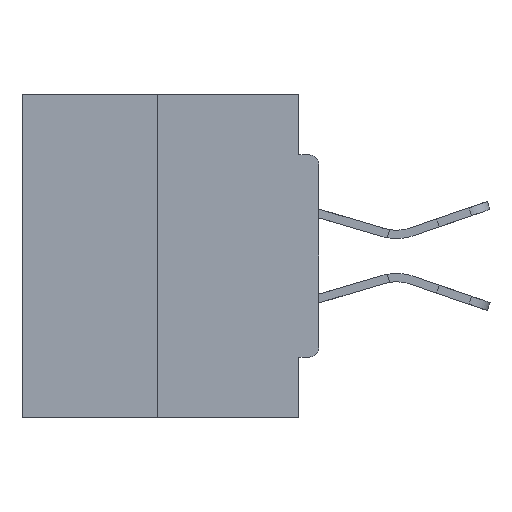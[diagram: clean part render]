
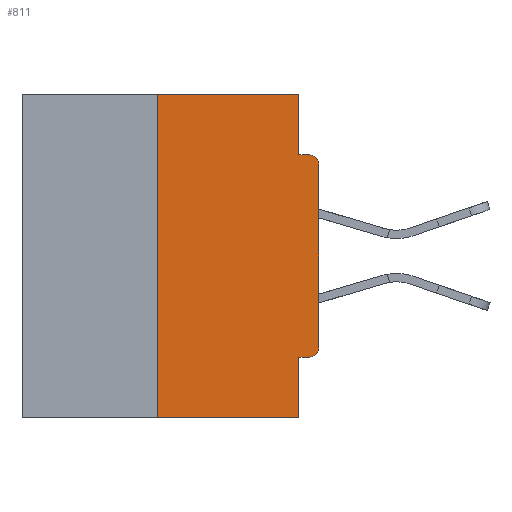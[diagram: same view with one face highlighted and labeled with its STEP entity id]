
A CAD part, left-side view. The second image highlights one B-rep face of the part: STEP entity #811.
In plain terms, the highlighted planar face has unit normal (-1, 0, 0).
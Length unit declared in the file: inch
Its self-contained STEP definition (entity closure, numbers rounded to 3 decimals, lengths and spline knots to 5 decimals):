
#811 = ADVANCED_FACE ( 'NONE', ( #11854 ), #10083, .F. ) ;
#915 = CARTESIAN_POINT ( 'NONE',  ( 0., 0.031, 0. ) ) ;
#2630 = AXIS2_PLACEMENT_3D ( 'NONE', #7279, #28383, #31005 ) ;
#3054 = LINE ( 'NONE', #5576, #21504 ) ;
#3866 = CARTESIAN_POINT ( 'NONE',  ( 0., 0.015, -0.4065 ) ) ;
#4381 = EDGE_CURVE ( 'NONE', #31245, #14231, #3054, .T. ) ;
#4686 = CARTESIAN_POINT ( 'NONE',  ( 0., 0.031, -0.4065 ) ) ;
#4790 = EDGE_CURVE ( 'NONE', #15706, #33267, #16122, .T. ) ;
#5576 = CARTESIAN_POINT ( 'NONE',  ( 0., 0., -0.0935 ) ) ;
#6225 = LINE ( 'NONE', #30858, #16854 ) ;
#6309 = DIRECTION ( 'NONE',  ( 0., 0., -1. ) ) ;
#6626 = DIRECTION ( 'NONE',  ( 0., -1., 0. ) ) ;
#7039 = VERTEX_POINT ( 'NONE', #24957 ) ;
#7138 = ORIENTED_EDGE ( 'NONE', *, *, #28937, .F. ) ;
#7237 = CARTESIAN_POINT ( 'NONE',  ( 0., 0.25, 0. ) ) ;
#7279 = CARTESIAN_POINT ( 'NONE',  ( 0., 0.015, -0.3915 ) ) ;
#7896 = DIRECTION ( 'NONE',  ( 0., 0., 1. ) ) ;
#8215 = VERTEX_POINT ( 'NONE', #30735 ) ;
#8433 = ORIENTED_EDGE ( 'NONE', *, *, #21307, .T. ) ;
#9488 = CARTESIAN_POINT ( 'NONE',  ( 0., 0.25, 0. ) ) ;
#9512 = VECTOR ( 'NONE', #22536, 39.37008 ) ;
#9720 = EDGE_CURVE ( 'NONE', #23108, #31245, #22672, .T. ) ;
#10083 = PLANE ( 'NONE',  #23533 ) ;
#10325 = CARTESIAN_POINT ( 'NONE',  ( 0., 0.015, -0.0935 ) ) ;
#10364 = DIRECTION ( 'NONE',  ( 0., -1., 0. ) ) ;
#11040 = ORIENTED_EDGE ( 'NONE', *, *, #19071, .T. ) ;
#11854 = FACE_OUTER_BOUND ( 'NONE', #15785, .T. ) ;
#12369 = DIRECTION ( 'NONE',  ( 0., 0., -1. ) ) ;
#13281 = VECTOR ( 'NONE', #18262, 39.37008 ) ;
#13799 = CARTESIAN_POINT ( 'NONE',  ( 0., 0., -0.1085 ) ) ;
#14213 = VERTEX_POINT ( 'NONE', #7237 ) ;
#14231 = VERTEX_POINT ( 'NONE', #10325 ) ;
#15110 = DIRECTION ( 'NONE',  ( 0., 0., -1. ) ) ;
#15706 = VERTEX_POINT ( 'NONE', #3866 ) ;
#15785 = EDGE_LOOP ( 'NONE', ( #24351, #17630, #11040, #7138, #28497, #24958, #16997, #8433, #25123, #32436 ) ) ;
#16122 = LINE ( 'NONE', #23552, #13281 ) ;
#16509 = CARTESIAN_POINT ( 'NONE',  ( 0., 0.015, -0.1085 ) ) ;
#16854 = VECTOR ( 'NONE', #15110, 39.37008 ) ;
#16997 = ORIENTED_EDGE ( 'NONE', *, *, #31982, .T. ) ;
#17535 = DIRECTION ( 'NONE',  ( 1., 0., 0. ) ) ;
#17630 = ORIENTED_EDGE ( 'NONE', *, *, #28107, .F. ) ;
#17719 = VECTOR ( 'NONE', #10364, 39.37008 ) ;
#18262 = DIRECTION ( 'NONE',  ( 0., 1., 0. ) ) ;
#19071 = EDGE_CURVE ( 'NONE', #27847, #7039, #24706, .T. ) ;
#19269 = DIRECTION ( 'NONE',  ( -1., 0., 0. ) ) ;
#20211 = EDGE_CURVE ( 'NONE', #14213, #23108, #24123, .T. ) ;
#20874 = VECTOR ( 'NONE', #6626, 39.37008 ) ;
#21179 = CARTESIAN_POINT ( 'NONE',  ( 0., 0.25, -0.5 ) ) ;
#21307 = EDGE_CURVE ( 'NONE', #25282, #14231, #23636, .T. ) ;
#21504 = VECTOR ( 'NONE', #26686, 39.37008 ) ;
#21807 = DIRECTION ( 'NONE',  ( 0., 0., -1. ) ) ;
#22213 = EDGE_CURVE ( 'NONE', #15706, #8215, #29349, .T. ) ;
#22536 = DIRECTION ( 'NONE',  ( 0., 0., 1. ) ) ;
#22672 = LINE ( 'NONE', #915, #28021 ) ;
#23108 = VERTEX_POINT ( 'NONE', #24574 ) ;
#23533 = AXIS2_PLACEMENT_3D ( 'NONE', #28099, #17535, #12369 ) ;
#23552 = CARTESIAN_POINT ( 'NONE',  ( 0., 0., -0.4065 ) ) ;
#23636 = CIRCLE ( 'NONE', #24374, 0.015 ) ;
#23660 = CARTESIAN_POINT ( 'NONE',  ( 0., 0.46, -0.5 ) ) ;
#23825 = LINE ( 'NONE', #9488, #9512 ) ;
#24123 = LINE ( 'NONE', #27152, #20874 ) ;
#24351 = ORIENTED_EDGE ( 'NONE', *, *, #20211, .F. ) ;
#24374 = AXIS2_PLACEMENT_3D ( 'NONE', #16509, #19269, #21807 ) ;
#24574 = CARTESIAN_POINT ( 'NONE',  ( 0., 0.031, 0. ) ) ;
#24706 = LINE ( 'NONE', #23660, #17719 ) ;
#24957 = CARTESIAN_POINT ( 'NONE',  ( 0., 0.031, -0.5 ) ) ;
#24958 = ORIENTED_EDGE ( 'NONE', *, *, #22213, .T. ) ;
#25123 = ORIENTED_EDGE ( 'NONE', *, *, #4381, .F. ) ;
#25282 = VERTEX_POINT ( 'NONE', #13799 ) ;
#26686 = DIRECTION ( 'NONE',  ( 0., -1., 0. ) ) ;
#27152 = CARTESIAN_POINT ( 'NONE',  ( 0., 0.46, 0. ) ) ;
#27847 = VERTEX_POINT ( 'NONE', #21179 ) ;
#28021 = VECTOR ( 'NONE', #6309, 39.37008 ) ;
#28099 = CARTESIAN_POINT ( 'NONE',  ( 0., 0.46, 0. ) ) ;
#28107 = EDGE_CURVE ( 'NONE', #27847, #14213, #23825, .T. ) ;
#28383 = DIRECTION ( 'NONE',  ( -1., 0., 0. ) ) ;
#28497 = ORIENTED_EDGE ( 'NONE', *, *, #4790, .F. ) ;
#28937 = EDGE_CURVE ( 'NONE', #33267, #7039, #6225, .T. ) ;
#29100 = CARTESIAN_POINT ( 'NONE',  ( 0., 0., 0. ) ) ;
#29349 = CIRCLE ( 'NONE', #2630, 0.015 ) ;
#30411 = CARTESIAN_POINT ( 'NONE',  ( 0., 0.031, -0.0935 ) ) ;
#30735 = CARTESIAN_POINT ( 'NONE',  ( 0., 0., -0.3915 ) ) ;
#30858 = CARTESIAN_POINT ( 'NONE',  ( 0., 0.031, -0.5 ) ) ;
#30976 = LINE ( 'NONE', #29100, #31816 ) ;
#31005 = DIRECTION ( 'NONE',  ( 0., 0., -1. ) ) ;
#31245 = VERTEX_POINT ( 'NONE', #30411 ) ;
#31816 = VECTOR ( 'NONE', #7896, 39.37008 ) ;
#31982 = EDGE_CURVE ( 'NONE', #8215, #25282, #30976, .T. ) ;
#32436 = ORIENTED_EDGE ( 'NONE', *, *, #9720, .F. ) ;
#33267 = VERTEX_POINT ( 'NONE', #4686 ) ;
